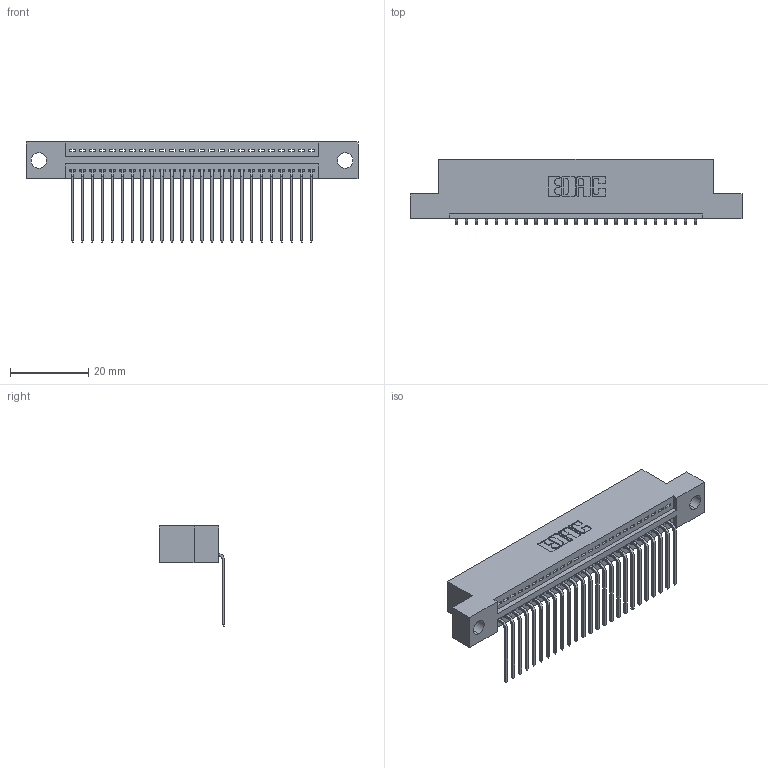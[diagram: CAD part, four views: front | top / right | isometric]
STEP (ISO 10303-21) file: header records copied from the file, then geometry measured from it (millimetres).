
FILE_DESCRIPTION (( 'STEP AP203' ), '1' );
FILE_NAME ('345-025-559-104.STEP', '2019-10-05T07:47:38', ( '' ), ( '' ), 'SwSTEP 2.0', 'SolidWorks 2016', '' );
FILE_SCHEMA (( 'CONFIG_CONTROL_DESIGN' ));
Length unit declared in the file: inch
Products named in the file (3): 345-292-001_558 559 Tail - 1; 345 Part_Flush Mounting Lugs - 0.156 Dia-TH; 345-025-559-104
Assembly tree (26 placements, depth 2):
  345-025-559-104
    345 Part_Flush Mounting Lugs - 0.156 Dia-TH
    345-292-001_558 559 Tail - 1  x25
Bounding box: 84.71 x 16.75 x 25.53 mm (x, y, z)
Volume: 7901.9 mm3; surface area: 10568.1 mm2
Topology: 26 solids, 26 shells, 1626 faces, 4891 edges, 3226 vertices
Faces by surface type: plane 1130, cylinder 496
Entity records: 21191 total; most frequent: CARTESIAN_POINT 3679, ORIENTED_EDGE 3638, DIRECTION 3237, EDGE_CURVE 1819, LINE 1587, VECTOR 1587, VERTEX_POINT 1210, AXIS2_PLACEMENT_3D 825
